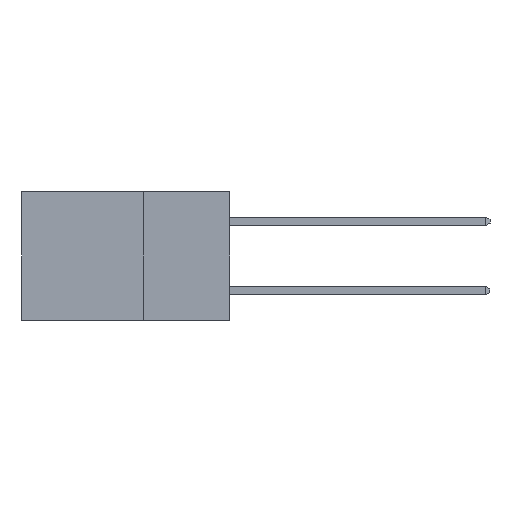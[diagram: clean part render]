
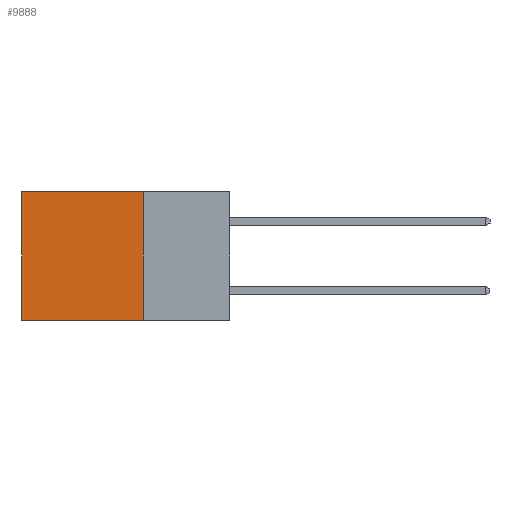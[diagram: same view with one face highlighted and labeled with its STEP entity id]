
A CAD part, left-side view. The second image highlights one B-rep face of the part: STEP entity #9888.
In plain terms, the highlighted planar face has unit normal (-1, 0, 0).
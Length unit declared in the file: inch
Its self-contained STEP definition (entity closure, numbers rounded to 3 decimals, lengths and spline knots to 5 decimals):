
#2200 = CARTESIAN_POINT ( 'NONE',  ( 0.298, 0.6, 0. ) ) ;
#2991 = AXIS2_PLACEMENT_3D ( 'NONE', #3180, #3112, #3108 ) ;
#3067 = VECTOR ( 'NONE', #7130, 39.37008 ) ;
#3108 = DIRECTION ( 'NONE',  ( 0., 0., -1. ) ) ;
#3112 = DIRECTION ( 'NONE',  ( 1., 0., 0. ) ) ;
#3180 = CARTESIAN_POINT ( 'NONE',  ( 0.298, 0.25, 0. ) ) ;
#3257 = ORIENTED_EDGE ( 'NONE', *, *, #12071, .F. ) ;
#3404 = PLANE ( 'NONE',  #2991 ) ;
#3500 = ORIENTED_EDGE ( 'NONE', *, *, #16587, .F. ) ;
#3680 = DIRECTION ( 'NONE',  ( 0., 0., -1. ) ) ;
#3922 = ORIENTED_EDGE ( 'NONE', *, *, #6456, .T. ) ;
#4685 = VERTEX_POINT ( 'NONE', #5358 ) ;
#5358 = CARTESIAN_POINT ( 'NONE',  ( 0.298, 0.6, -0.37 ) ) ;
#5544 = ORIENTED_EDGE ( 'NONE', *, *, #12933, .T. ) ;
#5564 = VERTEX_POINT ( 'NONE', #13983 ) ;
#6390 = CARTESIAN_POINT ( 'NONE',  ( 0.298, 0.25, 0. ) ) ;
#6456 = EDGE_CURVE ( 'NONE', #8290, #9203, #9446, .T. ) ;
#7130 = DIRECTION ( 'NONE',  ( 0., 0., -1. ) ) ;
#7615 = CARTESIAN_POINT ( 'NONE',  ( 0.298, 0.6, 0. ) ) ;
#8290 = VERTEX_POINT ( 'NONE', #6390 ) ;
#8470 = CARTESIAN_POINT ( 'NONE',  ( 0.298, 0.25, 0. ) ) ;
#8762 = VECTOR ( 'NONE', #3680, 39.37008 ) ;
#9203 = VERTEX_POINT ( 'NONE', #7615 ) ;
#9446 = LINE ( 'NONE', #14328, #12491 ) ;
#9888 = ADVANCED_FACE ( 'NONE', ( #16596 ), #3404, .F. ) ;
#10135 = CARTESIAN_POINT ( 'NONE',  ( 0.298, 0.25, -0.37 ) ) ;
#11496 = LINE ( 'NONE', #10135, #14019 ) ;
#12071 = EDGE_CURVE ( 'NONE', #8290, #5564, #16895, .T. ) ;
#12491 = VECTOR ( 'NONE', #14283, 39.37008 ) ;
#12933 = EDGE_CURVE ( 'NONE', #9203, #4685, #15547, .T. ) ;
#13956 = DIRECTION ( 'NONE',  ( 0., 1., 0. ) ) ;
#13983 = CARTESIAN_POINT ( 'NONE',  ( 0.298, 0.25, -0.37 ) ) ;
#14019 = VECTOR ( 'NONE', #13956, 39.37008 ) ;
#14283 = DIRECTION ( 'NONE',  ( 0., 1., 0. ) ) ;
#14328 = CARTESIAN_POINT ( 'NONE',  ( 0.298, 0.25, 0. ) ) ;
#14630 = EDGE_LOOP ( 'NONE', ( #5544, #3500, #3257, #3922 ) ) ;
#15547 = LINE ( 'NONE', #2200, #8762 ) ;
#16587 = EDGE_CURVE ( 'NONE', #5564, #4685, #11496, .T. ) ;
#16596 = FACE_OUTER_BOUND ( 'NONE', #14630, .T. ) ;
#16895 = LINE ( 'NONE', #8470, #3067 ) ;
